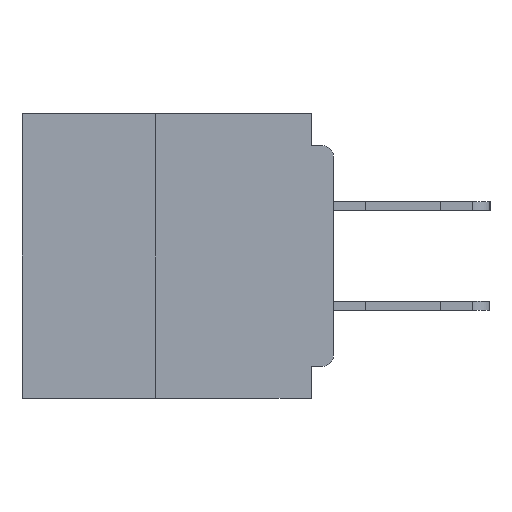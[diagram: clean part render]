
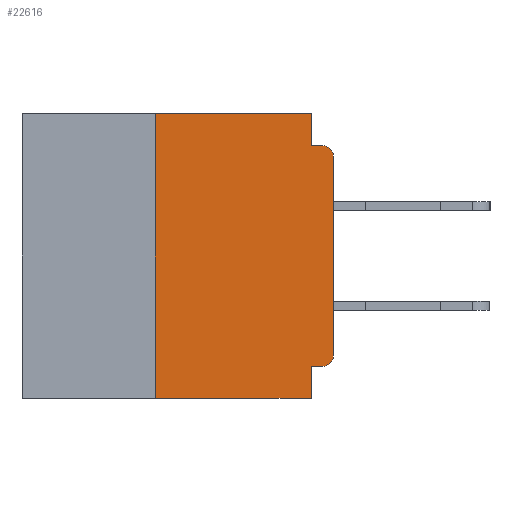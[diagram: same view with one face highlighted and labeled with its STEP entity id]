
A CAD part, left-side view. The second image highlights one B-rep face of the part: STEP entity #22616.
In plain terms, the highlighted planar face has unit normal (-1, 0, 0).
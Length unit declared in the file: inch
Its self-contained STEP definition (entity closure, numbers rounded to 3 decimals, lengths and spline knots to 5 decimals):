
#291 = DIRECTION ( 'NONE',  ( 0., 0., -1. ) ) ;
#1289 = EDGE_CURVE ( 'NONE', #13603, #15730, #22100, .T. ) ;
#2816 = ORIENTED_EDGE ( 'NONE', *, *, #1289, .T. ) ;
#3049 = DIRECTION ( 'NONE',  ( 0., 0., -1. ) ) ;
#4052 = VERTEX_POINT ( 'NONE', #46683 ) ;
#5352 = DIRECTION ( 'NONE',  ( 0., -1., 0. ) ) ;
#6297 = ORIENTED_EDGE ( 'NONE', *, *, #17699, .T. ) ;
#6691 = DIRECTION ( 'NONE',  ( 0., 0., 1. ) ) ;
#6853 = PLANE ( 'NONE',  #44245 ) ;
#7153 = VERTEX_POINT ( 'NONE', #35342 ) ;
#7670 = ORIENTED_EDGE ( 'NONE', *, *, #47509, .F. ) ;
#7833 = LINE ( 'NONE', #33219, #28800 ) ;
#8281 = AXIS2_PLACEMENT_3D ( 'NONE', #11327, #38842, #15293 ) ;
#8620 = FACE_OUTER_BOUND ( 'NONE', #15027, .T. ) ;
#9694 = EDGE_CURVE ( 'NONE', #13603, #4052, #44311, .T. ) ;
#10308 = LINE ( 'NONE', #23915, #31248 ) ;
#10433 = DIRECTION ( 'NONE',  ( 0., 0., -1. ) ) ;
#10666 = CARTESIAN_POINT ( 'NONE',  ( 0., 0.25, -0.4 ) ) ;
#11326 = VECTOR ( 'NONE', #6691, 39.37008 ) ;
#11327 = CARTESIAN_POINT ( 'NONE',  ( 0., 0.015, -0.06 ) ) ;
#11619 = ORIENTED_EDGE ( 'NONE', *, *, #9694, .F. ) ;
#12197 = LINE ( 'NONE', #34003, #13395 ) ;
#13395 = VECTOR ( 'NONE', #10433, 39.37008 ) ;
#13464 = CARTESIAN_POINT ( 'NONE',  ( 0., 0., -0.06 ) ) ;
#13516 = VERTEX_POINT ( 'NONE', #19192 ) ;
#13603 = VERTEX_POINT ( 'NONE', #15870 ) ;
#13684 = CARTESIAN_POINT ( 'NONE',  ( 0., 0.437, -0.4 ) ) ;
#13780 = ORIENTED_EDGE ( 'NONE', *, *, #43981, .F. ) ;
#14777 = CIRCLE ( 'NONE', #8281, 0.015 ) ;
#15027 = EDGE_LOOP ( 'NONE', ( #23774, #46728, #18136, #46359, #21568, #7670, #6297, #13780, #11619, #2816 ) ) ;
#15293 = DIRECTION ( 'NONE',  ( 0., 0., -1. ) ) ;
#15730 = VERTEX_POINT ( 'NONE', #41077 ) ;
#15870 = CARTESIAN_POINT ( 'NONE',  ( 0., 0.015, -0.355 ) ) ;
#17304 = EDGE_CURVE ( 'NONE', #33057, #13516, #14777, .T. ) ;
#17699 = EDGE_CURVE ( 'NONE', #44143, #31570, #18503, .T. ) ;
#17729 = DIRECTION ( 'NONE',  ( 0., -1., 0. ) ) ;
#18136 = ORIENTED_EDGE ( 'NONE', *, *, #30192, .F. ) ;
#18503 = LINE ( 'NONE', #13684, #36882 ) ;
#19192 = CARTESIAN_POINT ( 'NONE',  ( 0., 0.015, -0.045 ) ) ;
#19387 = CARTESIAN_POINT ( 'NONE',  ( 0., 0.031, -0.4 ) ) ;
#19436 = DIRECTION ( 'NONE',  ( 0., 1., 0. ) ) ;
#21568 = ORIENTED_EDGE ( 'NONE', *, *, #35005, .F. ) ;
#21606 = DIRECTION ( 'NONE',  ( 0., 0., 1. ) ) ;
#22100 = CIRCLE ( 'NONE', #37745, 0.015 ) ;
#22616 = ADVANCED_FACE ( 'NONE', ( #8620 ), #6853, .F. ) ;
#23240 = DIRECTION ( 'NONE',  ( 0., 0., -1. ) ) ;
#23303 = DIRECTION ( 'NONE',  ( -1., 0., 0. ) ) ;
#23572 = CARTESIAN_POINT ( 'NONE',  ( 0., 0.015, -0.34 ) ) ;
#23774 = ORIENTED_EDGE ( 'NONE', *, *, #24171, .T. ) ;
#23881 = CARTESIAN_POINT ( 'NONE',  ( 0., 0.437, 0. ) ) ;
#23915 = CARTESIAN_POINT ( 'NONE',  ( 0., 0.031, -0.4 ) ) ;
#24171 = EDGE_CURVE ( 'NONE', #15730, #33057, #7833, .T. ) ;
#25036 = CARTESIAN_POINT ( 'NONE',  ( 0., 0., -0.045 ) ) ;
#26670 = DIRECTION ( 'NONE',  ( 1., 0., 0. ) ) ;
#27828 = DIRECTION ( 'NONE',  ( 0., -1., 0. ) ) ;
#28800 = VECTOR ( 'NONE', #21606, 39.37008 ) ;
#28819 = VERTEX_POINT ( 'NONE', #31674 ) ;
#28962 = LINE ( 'NONE', #23881, #39368 ) ;
#29082 = LINE ( 'NONE', #25036, #48728 ) ;
#30192 = EDGE_CURVE ( 'NONE', #7153, #13516, #29082, .T. ) ;
#31248 = VECTOR ( 'NONE', #291, 39.37008 ) ;
#31570 = VERTEX_POINT ( 'NONE', #19387 ) ;
#31674 = CARTESIAN_POINT ( 'NONE',  ( 0., 0.25, 0. ) ) ;
#32272 = LINE ( 'NONE', #10666, #11326 ) ;
#32538 = EDGE_CURVE ( 'NONE', #50636, #7153, #12197, .T. ) ;
#32638 = VECTOR ( 'NONE', #19436, 39.37008 ) ;
#33057 = VERTEX_POINT ( 'NONE', #13464 ) ;
#33219 = CARTESIAN_POINT ( 'NONE',  ( 0., 0., 0. ) ) ;
#34003 = CARTESIAN_POINT ( 'NONE',  ( 0., 0.031, 0. ) ) ;
#35005 = EDGE_CURVE ( 'NONE', #28819, #50636, #28962, .T. ) ;
#35342 = CARTESIAN_POINT ( 'NONE',  ( 0., 0.031, -0.045 ) ) ;
#36882 = VECTOR ( 'NONE', #17729, 39.37008 ) ;
#37745 = AXIS2_PLACEMENT_3D ( 'NONE', #23572, #23303, #23240 ) ;
#38352 = CARTESIAN_POINT ( 'NONE',  ( 0., 0.437, 0. ) ) ;
#38842 = DIRECTION ( 'NONE',  ( -1., 0., 0. ) ) ;
#39368 = VECTOR ( 'NONE', #27828, 39.37008 ) ;
#41077 = CARTESIAN_POINT ( 'NONE',  ( 0., 0., -0.34 ) ) ;
#43981 = EDGE_CURVE ( 'NONE', #4052, #31570, #10308, .T. ) ;
#44143 = VERTEX_POINT ( 'NONE', #48263 ) ;
#44245 = AXIS2_PLACEMENT_3D ( 'NONE', #38352, #26670, #3049 ) ;
#44311 = LINE ( 'NONE', #50787, #32638 ) ;
#46359 = ORIENTED_EDGE ( 'NONE', *, *, #32538, .F. ) ;
#46683 = CARTESIAN_POINT ( 'NONE',  ( 0., 0.031, -0.355 ) ) ;
#46728 = ORIENTED_EDGE ( 'NONE', *, *, #17304, .T. ) ;
#47509 = EDGE_CURVE ( 'NONE', #44143, #28819, #32272, .T. ) ;
#48263 = CARTESIAN_POINT ( 'NONE',  ( 0., 0.25, -0.4 ) ) ;
#48728 = VECTOR ( 'NONE', #5352, 39.37008 ) ;
#49567 = CARTESIAN_POINT ( 'NONE',  ( 0., 0.031, 0. ) ) ;
#50636 = VERTEX_POINT ( 'NONE', #49567 ) ;
#50787 = CARTESIAN_POINT ( 'NONE',  ( 0., 0., -0.355 ) ) ;
